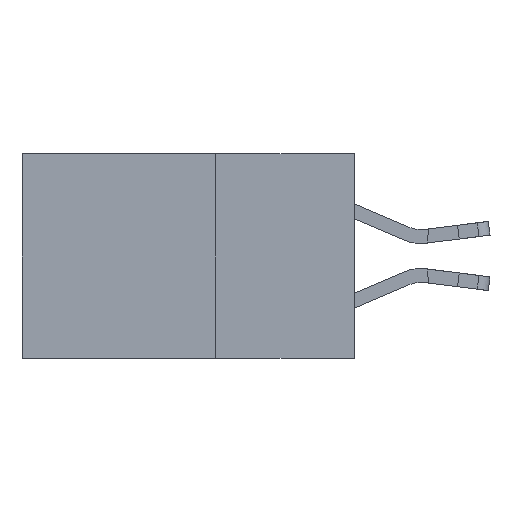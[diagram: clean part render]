
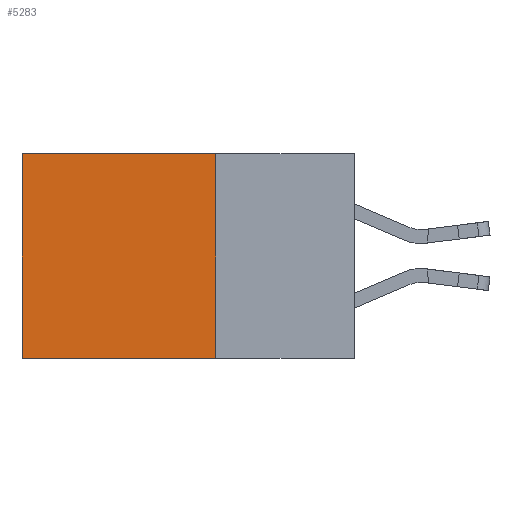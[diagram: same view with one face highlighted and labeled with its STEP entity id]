
A CAD part, left-side view. The second image highlights one B-rep face of the part: STEP entity #5283.
In plain terms, the highlighted planar face has unit normal (-1, 0, 0).
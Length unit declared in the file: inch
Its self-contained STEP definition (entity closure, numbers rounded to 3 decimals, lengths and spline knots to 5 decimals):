
#844 = DIRECTION ( 'NONE',  ( 0., 0., -1. ) ) ;
#1208 = FACE_OUTER_BOUND ( 'NONE', #10725, .T. ) ;
#1256 = ORIENTED_EDGE ( 'NONE', *, *, #4928, .T. ) ;
#2218 = CARTESIAN_POINT ( 'NONE',  ( 0.2615, 0.25, 0. ) ) ;
#2974 = LINE ( 'NONE', #11114, #3945 ) ;
#3231 = DIRECTION ( 'NONE',  ( 0., 1., 0. ) ) ;
#3879 = CARTESIAN_POINT ( 'NONE',  ( 0.2615, 0.25, 0. ) ) ;
#3945 = VECTOR ( 'NONE', #6181, 39.37008 ) ;
#4670 = AXIS2_PLACEMENT_3D ( 'NONE', #14603, #21319, #6258 ) ;
#4928 = EDGE_CURVE ( 'NONE', #5404, #6494, #2974, .T. ) ;
#5283 = ADVANCED_FACE ( 'NONE', ( #1208 ), #12953, .F. ) ;
#5404 = VERTEX_POINT ( 'NONE', #18435 ) ;
#6181 = DIRECTION ( 'NONE',  ( 0., 0., -1. ) ) ;
#6258 = DIRECTION ( 'NONE',  ( 0., 0., -1. ) ) ;
#6494 = VERTEX_POINT ( 'NONE', #13684 ) ;
#7019 = VERTEX_POINT ( 'NONE', #3879 ) ;
#7360 = EDGE_CURVE ( 'NONE', #7019, #5404, #13293, .T. ) ;
#7546 = LINE ( 'NONE', #15901, #20751 ) ;
#9286 = VECTOR ( 'NONE', #16696, 39.37008 ) ;
#10488 = VECTOR ( 'NONE', #3231, 39.37008 ) ;
#10725 = EDGE_LOOP ( 'NONE', ( #1256, #13989, #14081, #13214 ) ) ;
#11114 = CARTESIAN_POINT ( 'NONE',  ( 0.2615, 0.6, -0.37 ) ) ;
#11275 = CARTESIAN_POINT ( 'NONE',  ( 0.2615, 0.25, -0.37 ) ) ;
#12953 = PLANE ( 'NONE',  #4670 ) ;
#13214 = ORIENTED_EDGE ( 'NONE', *, *, #7360, .T. ) ;
#13293 = LINE ( 'NONE', #2218, #9286 ) ;
#13684 = CARTESIAN_POINT ( 'NONE',  ( 0.2615, 0.6, -0.37 ) ) ;
#13989 = ORIENTED_EDGE ( 'NONE', *, *, #18030, .F. ) ;
#14081 = ORIENTED_EDGE ( 'NONE', *, *, #20139, .F. ) ;
#14603 = CARTESIAN_POINT ( 'NONE',  ( 0.2615, 0.25, -0.37 ) ) ;
#15232 = VERTEX_POINT ( 'NONE', #20211 ) ;
#15901 = CARTESIAN_POINT ( 'NONE',  ( 0.2615, 0.25, -0.37 ) ) ;
#16696 = DIRECTION ( 'NONE',  ( 0., 1., 0. ) ) ;
#18030 = EDGE_CURVE ( 'NONE', #15232, #6494, #21610, .T. ) ;
#18435 = CARTESIAN_POINT ( 'NONE',  ( 0.2615, 0.6, 0. ) ) ;
#20139 = EDGE_CURVE ( 'NONE', #7019, #15232, #7546, .T. ) ;
#20211 = CARTESIAN_POINT ( 'NONE',  ( 0.2615, 0.25, -0.37 ) ) ;
#20751 = VECTOR ( 'NONE', #844, 39.37008 ) ;
#21319 = DIRECTION ( 'NONE',  ( 1., 0., 0. ) ) ;
#21610 = LINE ( 'NONE', #11275, #10488 ) ;
